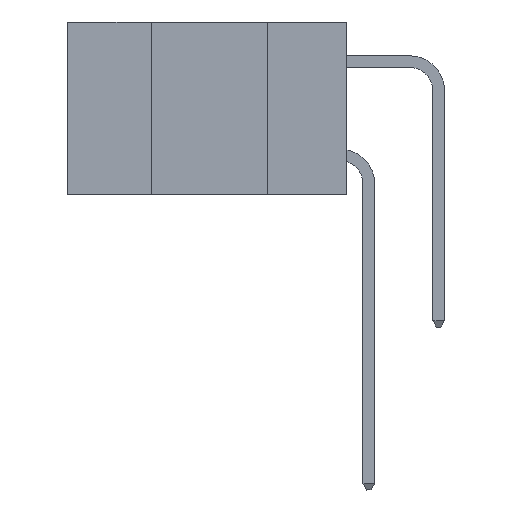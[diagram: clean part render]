
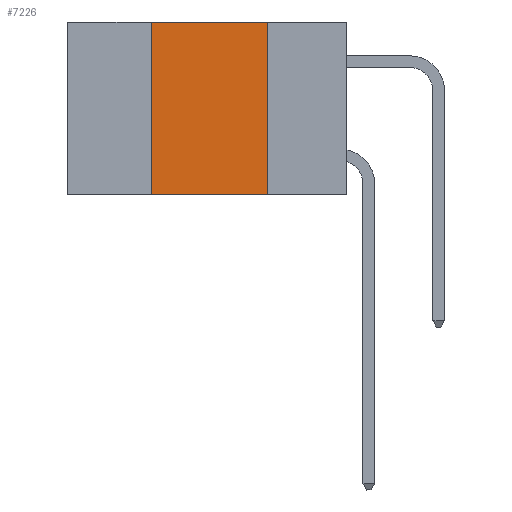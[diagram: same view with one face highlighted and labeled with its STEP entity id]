
A CAD part, left-side view. The second image highlights one B-rep face of the part: STEP entity #7226.
In plain terms, the highlighted planar face has unit normal (-1, 0, 0).
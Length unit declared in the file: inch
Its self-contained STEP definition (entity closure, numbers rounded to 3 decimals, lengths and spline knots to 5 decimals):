
#288 = CARTESIAN_POINT ( 'NONE',  ( 0., 0.6, 0. ) ) ;
#2530 = EDGE_CURVE ( 'NONE', #11256, #30244, #28047, .T. ) ;
#2925 = PLANE ( 'NONE',  #28638 ) ;
#6242 = DIRECTION ( 'NONE',  ( 1., 0., 0. ) ) ;
#7226 = ADVANCED_FACE ( 'NONE', ( #25394 ), #2925, .F. ) ;
#9705 = EDGE_CURVE ( 'NONE', #17772, #11256, #19529, .T. ) ;
#9716 = CARTESIAN_POINT ( 'NONE',  ( 0., 0.6, 0. ) ) ;
#11096 = VECTOR ( 'NONE', #13495, 39.37008 ) ;
#11256 = VERTEX_POINT ( 'NONE', #15185 ) ;
#13495 = DIRECTION ( 'NONE',  ( 0., -1., 0. ) ) ;
#13699 = VERTEX_POINT ( 'NONE', #16831 ) ;
#13808 = LINE ( 'NONE', #18742, #23644 ) ;
#15012 = DIRECTION ( 'NONE',  ( 0., 0., -1. ) ) ;
#15185 = CARTESIAN_POINT ( 'NONE',  ( 0., 0.42, 0. ) ) ;
#15652 = EDGE_CURVE ( 'NONE', #30244, #13699, #13808, .T. ) ;
#16831 = CARTESIAN_POINT ( 'NONE',  ( 0., 0.17, -0.37 ) ) ;
#17772 = VERTEX_POINT ( 'NONE', #23860 ) ;
#17831 = CARTESIAN_POINT ( 'NONE',  ( 0., 0.17, 0. ) ) ;
#18742 = CARTESIAN_POINT ( 'NONE',  ( 0., 0.17, 0. ) ) ;
#18959 = ORIENTED_EDGE ( 'NONE', *, *, #36356, .T. ) ;
#19529 = LINE ( 'NONE', #29890, #28769 ) ;
#19602 = ORIENTED_EDGE ( 'NONE', *, *, #2530, .F. ) ;
#21179 = VECTOR ( 'NONE', #26652, 39.37008 ) ;
#23224 = ORIENTED_EDGE ( 'NONE', *, *, #9705, .F. ) ;
#23644 = VECTOR ( 'NONE', #15012, 39.37008 ) ;
#23780 = ORIENTED_EDGE ( 'NONE', *, *, #15652, .F. ) ;
#23860 = CARTESIAN_POINT ( 'NONE',  ( 0., 0.42, -0.37 ) ) ;
#25394 = FACE_OUTER_BOUND ( 'NONE', #38557, .T. ) ;
#26085 = DIRECTION ( 'NONE',  ( 0., 0., -1. ) ) ;
#26652 = DIRECTION ( 'NONE',  ( 0., -1., 0. ) ) ;
#28047 = LINE ( 'NONE', #288, #11096 ) ;
#28638 = AXIS2_PLACEMENT_3D ( 'NONE', #9716, #6242, #26085 ) ;
#28769 = VECTOR ( 'NONE', #40206, 39.37008 ) ;
#29890 = CARTESIAN_POINT ( 'NONE',  ( 0., 0.42, 0. ) ) ;
#29918 = LINE ( 'NONE', #39421, #21179 ) ;
#30244 = VERTEX_POINT ( 'NONE', #17831 ) ;
#36356 = EDGE_CURVE ( 'NONE', #17772, #13699, #29918, .T. ) ;
#38557 = EDGE_LOOP ( 'NONE', ( #23780, #19602, #23224, #18959 ) ) ;
#39421 = CARTESIAN_POINT ( 'NONE',  ( 0., 0.6, -0.37 ) ) ;
#40206 = DIRECTION ( 'NONE',  ( 0., 0., 1. ) ) ;
